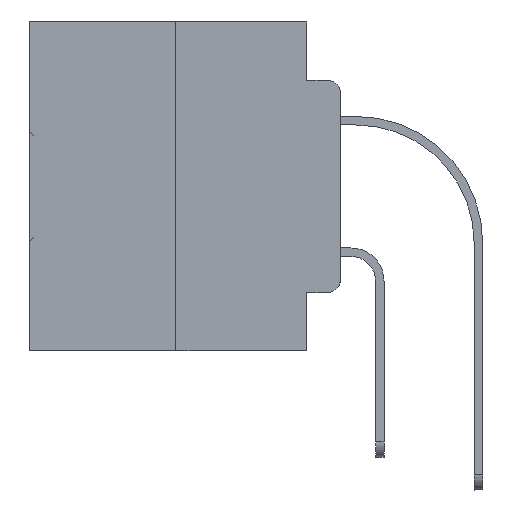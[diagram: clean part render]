
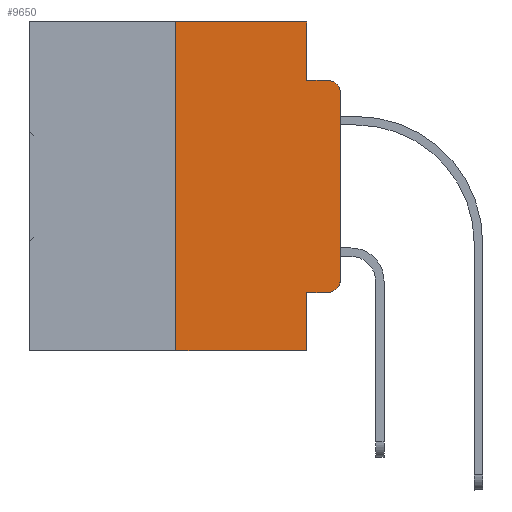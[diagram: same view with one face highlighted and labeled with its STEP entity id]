
A CAD part, left-side view. The second image highlights one B-rep face of the part: STEP entity #9650.
In plain terms, the highlighted planar face has unit normal (-1, 0, 0).
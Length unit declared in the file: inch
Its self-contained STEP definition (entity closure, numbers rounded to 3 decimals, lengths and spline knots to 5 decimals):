
#365 = VECTOR ( 'NONE', #8646, 39.37008 ) ;
#771 = VERTEX_POINT ( 'NONE', #20887 ) ;
#2211 = CARTESIAN_POINT ( 'NONE',  ( 0., 0.25, 0. ) ) ;
#2373 = EDGE_CURVE ( 'NONE', #33468, #771, #19908, .T. ) ;
#2722 = DIRECTION ( 'NONE',  ( 0., -1., 0. ) ) ;
#2744 = AXIS2_PLACEMENT_3D ( 'NONE', #5254, #5064, #16643 ) ;
#3028 = LINE ( 'NONE', #25823, #365 ) ;
#3975 = CARTESIAN_POINT ( 'NONE',  ( 0., 0., -0.3915 ) ) ;
#4058 = VECTOR ( 'NONE', #2722, 39.37008 ) ;
#4386 = VERTEX_POINT ( 'NONE', #27168 ) ;
#4505 = ORIENTED_EDGE ( 'NONE', *, *, #24758, .T. ) ;
#4899 = AXIS2_PLACEMENT_3D ( 'NONE', #29431, #10187, #24171 ) ;
#5064 = DIRECTION ( 'NONE',  ( 1., 0., 0. ) ) ;
#5254 = CARTESIAN_POINT ( 'NONE',  ( 0., 0.473, 0. ) ) ;
#6477 = ORIENTED_EDGE ( 'NONE', *, *, #14862, .T. ) ;
#6786 = VERTEX_POINT ( 'NONE', #2211 ) ;
#8011 = ORIENTED_EDGE ( 'NONE', *, *, #2373, .T. ) ;
#8202 = CARTESIAN_POINT ( 'NONE',  ( 0., 0.25, -0.5 ) ) ;
#8274 = CIRCLE ( 'NONE', #29151, 0.02 ) ;
#8646 = DIRECTION ( 'NONE',  ( 0., -1., 0. ) ) ;
#8759 = CARTESIAN_POINT ( 'NONE',  ( 0., 0.02, -0.1085 ) ) ;
#8924 = ORIENTED_EDGE ( 'NONE', *, *, #21555, .F. ) ;
#8988 = CARTESIAN_POINT ( 'NONE',  ( 0., 0.051, 0. ) ) ;
#9167 = DIRECTION ( 'NONE',  ( 0., 0., -1. ) ) ;
#9650 = ADVANCED_FACE ( 'NONE', ( #13858 ), #36655, .F. ) ;
#9905 = VECTOR ( 'NONE', #21753, 39.37008 ) ;
#10091 = CARTESIAN_POINT ( 'NONE',  ( 0., 0., 0. ) ) ;
#10187 = DIRECTION ( 'NONE',  ( -1., 0., 0. ) ) ;
#10379 = CARTESIAN_POINT ( 'NONE',  ( 0., 0.473, 0. ) ) ;
#12477 = VECTOR ( 'NONE', #21818, 39.37008 ) ;
#12699 = CARTESIAN_POINT ( 'NONE',  ( 0., 0., -0.1085 ) ) ;
#13858 = FACE_OUTER_BOUND ( 'NONE', #28495, .T. ) ;
#14738 = CARTESIAN_POINT ( 'NONE',  ( 0., 0.051, 0. ) ) ;
#14795 = ORIENTED_EDGE ( 'NONE', *, *, #17736, .F. ) ;
#14862 = EDGE_CURVE ( 'NONE', #22160, #36631, #8274, .T. ) ;
#15135 = LINE ( 'NONE', #8988, #21339 ) ;
#15216 = ORIENTED_EDGE ( 'NONE', *, *, #23346, .F. ) ;
#15546 = DIRECTION ( 'NONE',  ( -1., 0., 0. ) ) ;
#16180 = EDGE_CURVE ( 'NONE', #26277, #771, #22767, .T. ) ;
#16379 = CARTESIAN_POINT ( 'NONE',  ( 0., 0.473, -0.5 ) ) ;
#16643 = DIRECTION ( 'NONE',  ( 0., 0., -1. ) ) ;
#17736 = EDGE_CURVE ( 'NONE', #33468, #6786, #35439, .T. ) ;
#18401 = LINE ( 'NONE', #10379, #9905 ) ;
#19636 = CARTESIAN_POINT ( 'NONE',  ( 0., 0.051, 0. ) ) ;
#19908 = LINE ( 'NONE', #16379, #4058 ) ;
#20006 = VERTEX_POINT ( 'NONE', #19636 ) ;
#20203 = ORIENTED_EDGE ( 'NONE', *, *, #28210, .T. ) ;
#20509 = DIRECTION ( 'NONE',  ( 0., 0., -1. ) ) ;
#20887 = CARTESIAN_POINT ( 'NONE',  ( 0., 0.051, -0.5 ) ) ;
#21339 = VECTOR ( 'NONE', #9167, 39.37008 ) ;
#21555 = EDGE_CURVE ( 'NONE', #4386, #36631, #3028, .T. ) ;
#21753 = DIRECTION ( 'NONE',  ( 0., -1., 0. ) ) ;
#21818 = DIRECTION ( 'NONE',  ( 0., 0., 1. ) ) ;
#22045 = VECTOR ( 'NONE', #26133, 39.37008 ) ;
#22160 = VERTEX_POINT ( 'NONE', #12699 ) ;
#22767 = LINE ( 'NONE', #14738, #22045 ) ;
#23346 = EDGE_CURVE ( 'NONE', #20006, #4386, #15135, .T. ) ;
#23989 = CIRCLE ( 'NONE', #4899, 0.02 ) ;
#24171 = DIRECTION ( 'NONE',  ( 0., 0., -1. ) ) ;
#24591 = CARTESIAN_POINT ( 'NONE',  ( 0., 0.25, 0. ) ) ;
#24758 = EDGE_CURVE ( 'NONE', #29970, #22160, #35864, .T. ) ;
#25820 = ORIENTED_EDGE ( 'NONE', *, *, #35216, .T. ) ;
#25823 = CARTESIAN_POINT ( 'NONE',  ( 0., 0.051, -0.0885 ) ) ;
#26095 = VERTEX_POINT ( 'NONE', #35306 ) ;
#26133 = DIRECTION ( 'NONE',  ( 0., 0., -1. ) ) ;
#26185 = DIRECTION ( 'NONE',  ( 0., -1., 0. ) ) ;
#26277 = VERTEX_POINT ( 'NONE', #33784 ) ;
#27035 = DIRECTION ( 'NONE',  ( 0., 0., 1. ) ) ;
#27168 = CARTESIAN_POINT ( 'NONE',  ( 0., 0.051, -0.0885 ) ) ;
#28128 = CARTESIAN_POINT ( 'NONE',  ( 0., 0.051, -0.4115 ) ) ;
#28210 = EDGE_CURVE ( 'NONE', #26095, #29970, #23989, .T. ) ;
#28495 = EDGE_LOOP ( 'NONE', ( #4505, #6477, #8924, #15216, #29222, #14795, #8011, #30226, #25820, #20203 ) ) ;
#29151 = AXIS2_PLACEMENT_3D ( 'NONE', #8759, #15546, #20509 ) ;
#29222 = ORIENTED_EDGE ( 'NONE', *, *, #35123, .F. ) ;
#29431 = CARTESIAN_POINT ( 'NONE',  ( 0., 0.02, -0.3915 ) ) ;
#29970 = VERTEX_POINT ( 'NONE', #3975 ) ;
#30226 = ORIENTED_EDGE ( 'NONE', *, *, #16180, .F. ) ;
#30918 = LINE ( 'NONE', #28128, #31390 ) ;
#31390 = VECTOR ( 'NONE', #26185, 39.37008 ) ;
#33385 = VECTOR ( 'NONE', #27035, 39.37008 ) ;
#33468 = VERTEX_POINT ( 'NONE', #8202 ) ;
#33784 = CARTESIAN_POINT ( 'NONE',  ( 0., 0.051, -0.4115 ) ) ;
#35123 = EDGE_CURVE ( 'NONE', #6786, #20006, #18401, .T. ) ;
#35216 = EDGE_CURVE ( 'NONE', #26277, #26095, #30918, .T. ) ;
#35306 = CARTESIAN_POINT ( 'NONE',  ( 0., 0.02, -0.4115 ) ) ;
#35439 = LINE ( 'NONE', #24591, #33385 ) ;
#35864 = LINE ( 'NONE', #10091, #12477 ) ;
#36547 = CARTESIAN_POINT ( 'NONE',  ( 0., 0.02, -0.0885 ) ) ;
#36631 = VERTEX_POINT ( 'NONE', #36547 ) ;
#36655 = PLANE ( 'NONE',  #2744 ) ;
